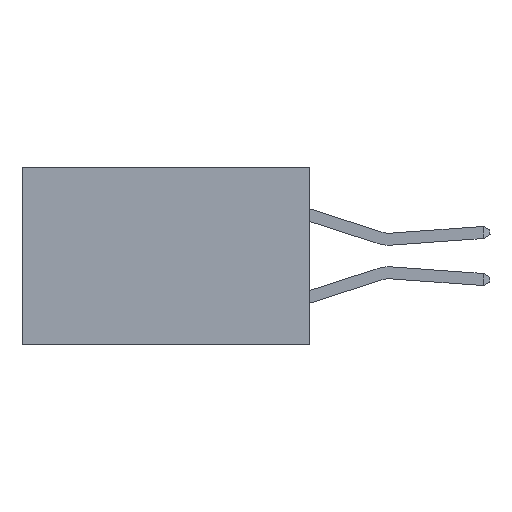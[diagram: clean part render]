
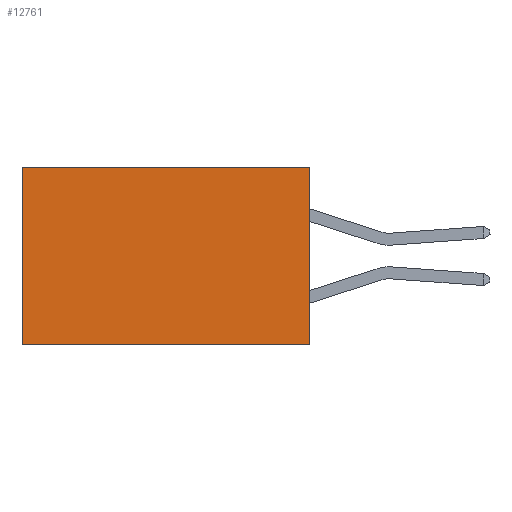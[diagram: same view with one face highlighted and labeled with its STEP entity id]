
A CAD part, left-side view. The second image highlights one B-rep face of the part: STEP entity #12761.
In plain terms, the highlighted planar face has unit normal (-1, 0, 0).
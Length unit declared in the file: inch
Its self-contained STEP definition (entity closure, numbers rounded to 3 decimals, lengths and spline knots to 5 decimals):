
#1245 = CARTESIAN_POINT ( 'NONE',  ( 0.2615, 0., 0. ) ) ;
#1471 = CARTESIAN_POINT ( 'NONE',  ( 0.2615, 0., -0.37 ) ) ;
#1871 = DIRECTION ( 'NONE',  ( 0., 0., -1. ) ) ;
#1915 = EDGE_LOOP ( 'NONE', ( #14733, #2863, #12359, #19228 ) ) ;
#2863 = ORIENTED_EDGE ( 'NONE', *, *, #15468, .F. ) ;
#2866 = LINE ( 'NONE', #1245, #12540 ) ;
#2980 = VERTEX_POINT ( 'NONE', #10405 ) ;
#4905 = DIRECTION ( 'NONE',  ( 0., 1., 0. ) ) ;
#5796 = LINE ( 'NONE', #7971, #22651 ) ;
#6657 = VECTOR ( 'NONE', #20559, 39.37008 ) ;
#7391 = VECTOR ( 'NONE', #1871, 39.37008 ) ;
#7971 = CARTESIAN_POINT ( 'NONE',  ( 0.2615, 0.6, -0.37 ) ) ;
#8094 = EDGE_CURVE ( 'NONE', #2980, #22491, #2866, .T. ) ;
#9353 = VERTEX_POINT ( 'NONE', #13501 ) ;
#10015 = DIRECTION ( 'NONE',  ( 0., 0., -1. ) ) ;
#10324 = CARTESIAN_POINT ( 'NONE',  ( 0.2615, 0., -0.37 ) ) ;
#10405 = CARTESIAN_POINT ( 'NONE',  ( 0.2615, 0., 0. ) ) ;
#12343 = EDGE_CURVE ( 'NONE', #2980, #24439, #20500, .T. ) ;
#12359 = ORIENTED_EDGE ( 'NONE', *, *, #12343, .F. ) ;
#12540 = VECTOR ( 'NONE', #4905, 39.37008 ) ;
#12761 = ADVANCED_FACE ( 'NONE', ( #14967 ), #13055, .F. ) ;
#12914 = DIRECTION ( 'NONE',  ( 0., 0., -1. ) ) ;
#13055 = PLANE ( 'NONE',  #24828 ) ;
#13501 = CARTESIAN_POINT ( 'NONE',  ( 0.2615, 0.6, -0.37 ) ) ;
#14237 = CARTESIAN_POINT ( 'NONE',  ( 0.2615, 0., -0.37 ) ) ;
#14733 = ORIENTED_EDGE ( 'NONE', *, *, #26508, .T. ) ;
#14967 = FACE_OUTER_BOUND ( 'NONE', #1915, .T. ) ;
#15468 = EDGE_CURVE ( 'NONE', #24439, #9353, #16053, .T. ) ;
#16053 = LINE ( 'NONE', #10324, #6657 ) ;
#19060 = DIRECTION ( 'NONE',  ( 1., 0., 0. ) ) ;
#19228 = ORIENTED_EDGE ( 'NONE', *, *, #8094, .T. ) ;
#20470 = CARTESIAN_POINT ( 'NONE',  ( 0.2615, 0., -0.37 ) ) ;
#20500 = LINE ( 'NONE', #14237, #7391 ) ;
#20559 = DIRECTION ( 'NONE',  ( 0., 1., 0. ) ) ;
#22491 = VERTEX_POINT ( 'NONE', #25970 ) ;
#22651 = VECTOR ( 'NONE', #10015, 39.37008 ) ;
#24439 = VERTEX_POINT ( 'NONE', #1471 ) ;
#24828 = AXIS2_PLACEMENT_3D ( 'NONE', #20470, #19060, #12914 ) ;
#25970 = CARTESIAN_POINT ( 'NONE',  ( 0.2615, 0.6, 0. ) ) ;
#26508 = EDGE_CURVE ( 'NONE', #22491, #9353, #5796, .T. ) ;
